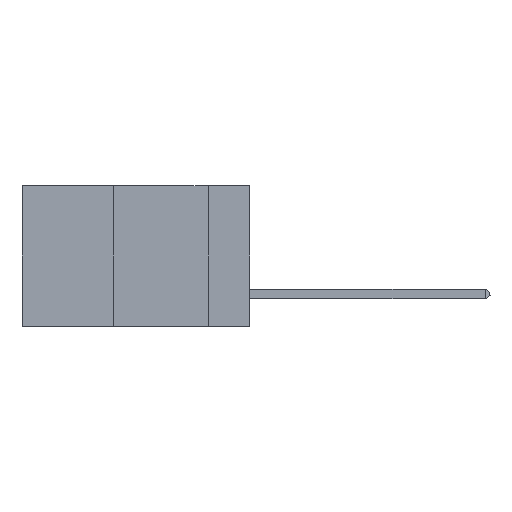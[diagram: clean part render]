
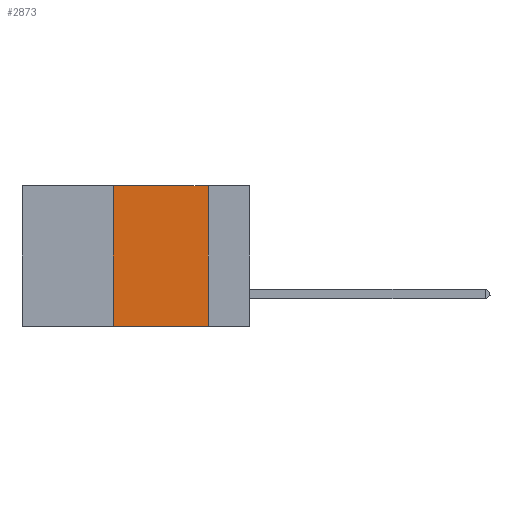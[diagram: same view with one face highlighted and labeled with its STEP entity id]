
A CAD part, left-side view. The second image highlights one B-rep face of the part: STEP entity #2873.
In plain terms, the highlighted planar face has unit normal (-1, 0, 0).
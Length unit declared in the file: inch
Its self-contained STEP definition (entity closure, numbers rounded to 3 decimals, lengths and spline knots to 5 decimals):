
#238 = DIRECTION ( 'NONE',  ( 0., -1., 0. ) ) ;
#358 = LINE ( 'NONE', #11075, #12442 ) ;
#762 = VECTOR ( 'NONE', #238, 39.37008 ) ;
#1694 = EDGE_CURVE ( 'NONE', #8776, #12427, #5666, .T. ) ;
#2534 = EDGE_CURVE ( 'NONE', #12427, #13676, #7594, .T. ) ;
#2873 = ADVANCED_FACE ( 'NONE', ( #5612 ), #12540, .F. ) ;
#3111 = CARTESIAN_POINT ( 'NONE',  ( 0., 0.36, 0. ) ) ;
#3433 = EDGE_CURVE ( 'NONE', #8776, #17977, #13486, .T. ) ;
#4774 = CARTESIAN_POINT ( 'NONE',  ( 0., 0.36, -0.37 ) ) ;
#4918 = CARTESIAN_POINT ( 'NONE',  ( 0., 0.11, -0.37 ) ) ;
#5384 = ORIENTED_EDGE ( 'NONE', *, *, #3433, .T. ) ;
#5511 = DIRECTION ( 'NONE',  ( 0., 0., -1. ) ) ;
#5612 = FACE_OUTER_BOUND ( 'NONE', #5759, .T. ) ;
#5666 = LINE ( 'NONE', #7064, #16193 ) ;
#5759 = EDGE_LOOP ( 'NONE', ( #16647, #14069, #12888, #5384 ) ) ;
#5969 = CARTESIAN_POINT ( 'NONE',  ( 0., 0.6, 0. ) ) ;
#7064 = CARTESIAN_POINT ( 'NONE',  ( 0., 0.36, 0. ) ) ;
#7085 = CARTESIAN_POINT ( 'NONE',  ( 0., 0.6, 0. ) ) ;
#7112 = VECTOR ( 'NONE', #14610, 39.37008 ) ;
#7594 = LINE ( 'NONE', #5969, #762 ) ;
#8776 = VERTEX_POINT ( 'NONE', #4774 ) ;
#11075 = CARTESIAN_POINT ( 'NONE',  ( 0., 0.11, 0. ) ) ;
#12191 = AXIS2_PLACEMENT_3D ( 'NONE', #7085, #13905, #16917 ) ;
#12427 = VERTEX_POINT ( 'NONE', #3111 ) ;
#12442 = VECTOR ( 'NONE', #5511, 39.37008 ) ;
#12540 = PLANE ( 'NONE',  #12191 ) ;
#12888 = ORIENTED_EDGE ( 'NONE', *, *, #1694, .F. ) ;
#13486 = LINE ( 'NONE', #14784, #7112 ) ;
#13676 = VERTEX_POINT ( 'NONE', #17824 ) ;
#13847 = EDGE_CURVE ( 'NONE', #13676, #17977, #358, .T. ) ;
#13905 = DIRECTION ( 'NONE',  ( 1., 0., 0. ) ) ;
#14069 = ORIENTED_EDGE ( 'NONE', *, *, #2534, .F. ) ;
#14610 = DIRECTION ( 'NONE',  ( 0., -1., 0. ) ) ;
#14784 = CARTESIAN_POINT ( 'NONE',  ( 0., 0.6, -0.37 ) ) ;
#15554 = DIRECTION ( 'NONE',  ( 0., 0., 1. ) ) ;
#16193 = VECTOR ( 'NONE', #15554, 39.37008 ) ;
#16647 = ORIENTED_EDGE ( 'NONE', *, *, #13847, .F. ) ;
#16917 = DIRECTION ( 'NONE',  ( 0., 0., -1. ) ) ;
#17824 = CARTESIAN_POINT ( 'NONE',  ( 0., 0.11, 0. ) ) ;
#17977 = VERTEX_POINT ( 'NONE', #4918 ) ;
